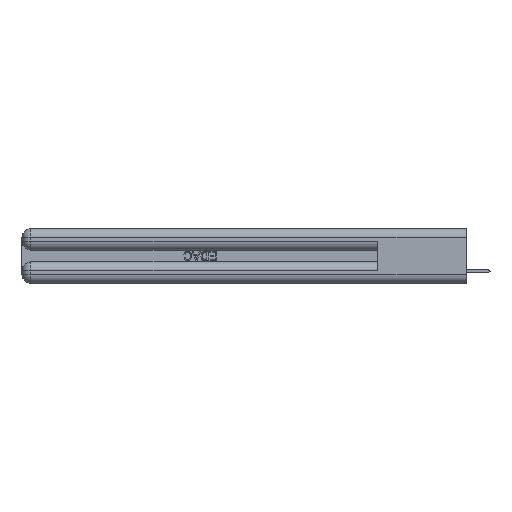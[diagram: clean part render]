
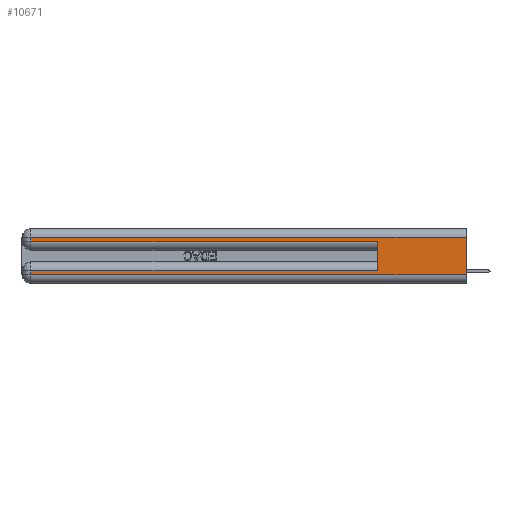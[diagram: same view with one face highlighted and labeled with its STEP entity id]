
A CAD part, left-side view. The second image highlights one B-rep face of the part: STEP entity #10671.
In plain terms, the highlighted planar face has unit normal (-1, 0, 0).
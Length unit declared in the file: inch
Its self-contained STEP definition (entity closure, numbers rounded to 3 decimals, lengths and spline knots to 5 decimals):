
#255 = VERTEX_POINT ( 'NONE', #816 ) ;
#816 = CARTESIAN_POINT ( 'NONE',  ( 0., 2.94, 0.06 ) ) ;
#2337 = LINE ( 'NONE', #47151, #5803 ) ;
#2514 = DIRECTION ( 'NONE',  ( 0., 0., -1. ) ) ;
#4032 = VECTOR ( 'NONE', #45303, 39.37008 ) ;
#4142 = EDGE_LOOP ( 'NONE', ( #12251, #24318, #12707, #28896, #22515, #11110, #34815, #38208 ) ) ;
#5803 = VECTOR ( 'NONE', #10541, 39.37008 ) ;
#6027 = DIRECTION ( 'NONE',  ( 1., 0., 0. ) ) ;
#7284 = EDGE_CURVE ( 'NONE', #32870, #12846, #41834, .T. ) ;
#7617 = CARTESIAN_POINT ( 'NONE',  ( 0., 0.6, 0.285 ) ) ;
#7879 = EDGE_CURVE ( 'NONE', #14137, #32870, #18324, .T. ) ;
#8424 = EDGE_CURVE ( 'NONE', #31367, #14137, #16167, .T. ) ;
#10541 = DIRECTION ( 'NONE',  ( 0., 0., -1. ) ) ;
#10671 = ADVANCED_FACE ( 'NONE', ( #23437 ), #35469, .F. ) ;
#11110 = ORIENTED_EDGE ( 'NONE', *, *, #27980, .T. ) ;
#11286 = VECTOR ( 'NONE', #36218, 39.37008 ) ;
#12251 = ORIENTED_EDGE ( 'NONE', *, *, #35538, .F. ) ;
#12707 = ORIENTED_EDGE ( 'NONE', *, *, #7879, .T. ) ;
#12846 = VERTEX_POINT ( 'NONE', #7617 ) ;
#13576 = CARTESIAN_POINT ( 'NONE',  ( 0., 0., 0.37 ) ) ;
#14137 = VERTEX_POINT ( 'NONE', #21704 ) ;
#14215 = CARTESIAN_POINT ( 'NONE',  ( 0., 0.6, 0.085 ) ) ;
#14681 = CARTESIAN_POINT ( 'NONE',  ( 0., 0., 0.06 ) ) ;
#15287 = CARTESIAN_POINT ( 'NONE',  ( 0., 2.94, 0.285 ) ) ;
#15642 = EDGE_CURVE ( 'NONE', #25648, #12846, #30094, .T. ) ;
#15660 = CARTESIAN_POINT ( 'NONE',  ( 0., 2.94, 0.37 ) ) ;
#16056 = VECTOR ( 'NONE', #17848, 39.37008 ) ;
#16121 = CARTESIAN_POINT ( 'NONE',  ( 0., 0., 0.31 ) ) ;
#16167 = LINE ( 'NONE', #36223, #34471 ) ;
#16333 = VERTEX_POINT ( 'NONE', #14681 ) ;
#16532 = CARTESIAN_POINT ( 'NONE',  ( 0., 0., 0.06 ) ) ;
#17284 = CARTESIAN_POINT ( 'NONE',  ( 0., 2.94, 0.37 ) ) ;
#17508 = AXIS2_PLACEMENT_3D ( 'NONE', #13576, #6027, #38972 ) ;
#17848 = DIRECTION ( 'NONE',  ( 0., -1., 0. ) ) ;
#17970 = CARTESIAN_POINT ( 'NONE',  ( 0., 0., 0.285 ) ) ;
#18324 = LINE ( 'NONE', #17284, #30803 ) ;
#19543 = EDGE_CURVE ( 'NONE', #255, #16333, #29744, .T. ) ;
#19883 = CARTESIAN_POINT ( 'NONE',  ( 0., 2.94, 0.085 ) ) ;
#20385 = CARTESIAN_POINT ( 'NONE',  ( 0., 0., 0.085 ) ) ;
#21704 = CARTESIAN_POINT ( 'NONE',  ( 0., 2.94, 0.31 ) ) ;
#21784 = CARTESIAN_POINT ( 'NONE',  ( 0., 0.6, 0.145 ) ) ;
#22515 = ORIENTED_EDGE ( 'NONE', *, *, #15642, .F. ) ;
#23437 = FACE_OUTER_BOUND ( 'NONE', #4142, .T. ) ;
#24076 = EDGE_CURVE ( 'NONE', #28819, #255, #34947, .T. ) ;
#24318 = ORIENTED_EDGE ( 'NONE', *, *, #8424, .T. ) ;
#25648 = VERTEX_POINT ( 'NONE', #14215 ) ;
#27980 = EDGE_CURVE ( 'NONE', #25648, #28819, #43736, .T. ) ;
#28819 = VERTEX_POINT ( 'NONE', #19883 ) ;
#28896 = ORIENTED_EDGE ( 'NONE', *, *, #7284, .T. ) ;
#29115 = DIRECTION ( 'NONE',  ( 0., 1., 0. ) ) ;
#29224 = DIRECTION ( 'NONE',  ( 0., -1., 0. ) ) ;
#29744 = LINE ( 'NONE', #16532, #16056 ) ;
#30094 = LINE ( 'NONE', #21784, #11286 ) ;
#30803 = VECTOR ( 'NONE', #2514, 39.37008 ) ;
#31367 = VERTEX_POINT ( 'NONE', #16121 ) ;
#32810 = VECTOR ( 'NONE', #37282, 39.37008 ) ;
#32870 = VERTEX_POINT ( 'NONE', #15287 ) ;
#34471 = VECTOR ( 'NONE', #29115, 39.37008 ) ;
#34815 = ORIENTED_EDGE ( 'NONE', *, *, #24076, .T. ) ;
#34947 = LINE ( 'NONE', #15660, #4032 ) ;
#35469 = PLANE ( 'NONE',  #17508 ) ;
#35538 = EDGE_CURVE ( 'NONE', #31367, #16333, #2337, .T. ) ;
#36218 = DIRECTION ( 'NONE',  ( 0., 0., 1. ) ) ;
#36223 = CARTESIAN_POINT ( 'NONE',  ( 0., 0., 0.31 ) ) ;
#37282 = DIRECTION ( 'NONE',  ( 0., 1., 0. ) ) ;
#38208 = ORIENTED_EDGE ( 'NONE', *, *, #19543, .T. ) ;
#38972 = DIRECTION ( 'NONE',  ( 0., 0., -1. ) ) ;
#41834 = LINE ( 'NONE', #17970, #43599 ) ;
#43599 = VECTOR ( 'NONE', #29224, 39.37008 ) ;
#43736 = LINE ( 'NONE', #20385, #32810 ) ;
#45303 = DIRECTION ( 'NONE',  ( 0., 0., -1. ) ) ;
#47151 = CARTESIAN_POINT ( 'NONE',  ( 0., 0., 0.37 ) ) ;
